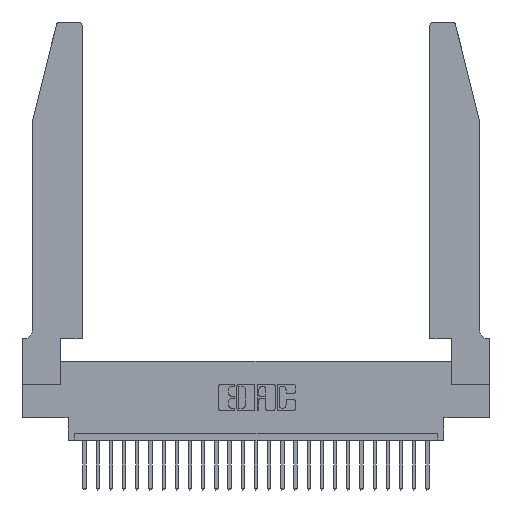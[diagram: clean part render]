
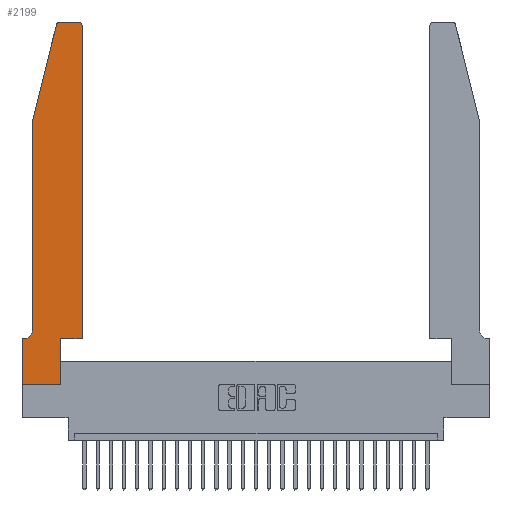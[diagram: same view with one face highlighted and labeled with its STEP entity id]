
A CAD part, top view. The second image highlights one B-rep face of the part: STEP entity #2199.
In plain terms, the highlighted planar face has unit normal (0, 0, 1).
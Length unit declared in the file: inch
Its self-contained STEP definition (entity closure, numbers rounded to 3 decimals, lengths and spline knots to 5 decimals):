
#155 = DIRECTION ( 'NONE',  ( 0., -1., 0. ) ) ;
#509 = VERTEX_POINT ( 'NONE', #19501 ) ;
#554 = CARTESIAN_POINT ( 'NONE',  ( 0., 0., 0.37 ) ) ;
#680 = DIRECTION ( 'NONE',  ( 1., 0., 0. ) ) ;
#775 = CARTESIAN_POINT ( 'NONE',  ( 0.4205, 2.72, 0.37 ) ) ;
#972 = VERTEX_POINT ( 'NONE', #25046 ) ;
#995 = ORIENTED_EDGE ( 'NONE', *, *, #1489, .T. ) ;
#1018 = LINE ( 'NONE', #25897, #25701 ) ;
#1271 = EDGE_CURVE ( 'NONE', #7114, #4585, #18498, .T. ) ;
#1489 = EDGE_CURVE ( 'NONE', #16377, #7114, #5650, .T. ) ;
#1569 = DIRECTION ( 'NONE',  ( -1., 0., 0. ) ) ;
#2199 = ADVANCED_FACE ( 'NONE', ( #20434 ), #17067, .T. ) ;
#2354 = CARTESIAN_POINT ( 'NONE',  ( 0.284, 2.75, 0.37 ) ) ;
#2361 = EDGE_CURVE ( 'NONE', #26980, #21348, #1018, .T. ) ;
#2566 = VECTOR ( 'NONE', #2654, 39.37008 ) ;
#2654 = DIRECTION ( 'NONE',  ( 1., 0., 0. ) ) ;
#2806 = DIRECTION ( 'NONE',  ( -0.239, -0.971, 0. ) ) ;
#2862 = EDGE_LOOP ( 'NONE', ( #25732, #5754, #26918, #20653, #3659, #995, #18751, #20708, #6925, #7870, #15923, #7170 ) ) ;
#2905 = CARTESIAN_POINT ( 'NONE',  ( 0.2865, 0.35, 0.37 ) ) ;
#2944 = DIRECTION ( 'NONE',  ( -1., 0., 0. ) ) ;
#3008 = VECTOR ( 'NONE', #6238, 39.37008 ) ;
#3348 = DIRECTION ( 'NONE',  ( 1., 0., 0. ) ) ;
#3659 = ORIENTED_EDGE ( 'NONE', *, *, #20299, .T. ) ;
#3690 = VECTOR ( 'NONE', #21560, 39.37008 ) ;
#4336 = CIRCLE ( 'NONE', #18900, 0.07 ) ;
#4585 = VERTEX_POINT ( 'NONE', #6536 ) ;
#4648 = VERTEX_POINT ( 'NONE', #2354 ) ;
#5087 = CARTESIAN_POINT ( 'NONE',  ( 0.0755, 0.42, 0.37 ) ) ;
#5310 = LINE ( 'NONE', #16421, #14200 ) ;
#5650 = LINE ( 'NONE', #9894, #16191 ) ;
#5754 = ORIENTED_EDGE ( 'NONE', *, *, #26614, .T. ) ;
#5980 = LINE ( 'NONE', #7974, #21845 ) ;
#6238 = DIRECTION ( 'NONE',  ( 0., 1., 0. ) ) ;
#6536 = CARTESIAN_POINT ( 'NONE',  ( 0., 0., 0.37 ) ) ;
#6803 = CARTESIAN_POINT ( 'NONE',  ( 0., 0., 0.37 ) ) ;
#6925 = ORIENTED_EDGE ( 'NONE', *, *, #19256, .T. ) ;
#7114 = VERTEX_POINT ( 'NONE', #18853 ) ;
#7170 = ORIENTED_EDGE ( 'NONE', *, *, #22832, .T. ) ;
#7190 = CARTESIAN_POINT ( 'NONE',  ( 0.4205, 2.75, 0.37 ) ) ;
#7447 = DIRECTION ( 'NONE',  ( 0., 0., 1. ) ) ;
#7870 = ORIENTED_EDGE ( 'NONE', *, *, #17607, .T. ) ;
#7974 = CARTESIAN_POINT ( 'NONE',  ( 0.2605, 2.75, 0.37 ) ) ;
#8051 = VERTEX_POINT ( 'NONE', #24405 ) ;
#9242 = DIRECTION ( 'NONE',  ( 0., 1., 0. ) ) ;
#9410 = EDGE_CURVE ( 'NONE', #21348, #13833, #5310, .T. ) ;
#9644 = VERTEX_POINT ( 'NONE', #16346 ) ;
#9894 = CARTESIAN_POINT ( 'NONE',  ( 0.0755, 0.35, 0.37 ) ) ;
#10034 = AXIS2_PLACEMENT_3D ( 'NONE', #14746, #19179, #21119 ) ;
#10352 = CARTESIAN_POINT ( 'NONE',  ( 0.25487, 2.72718, 0.37 ) ) ;
#10567 = CARTESIAN_POINT ( 'NONE',  ( 0.4505, 0.35, 0.37 ) ) ;
#10781 = CIRCLE ( 'NONE', #16338, 0.03 ) ;
#12180 = DIRECTION ( 'NONE',  ( -1., 0., 0. ) ) ;
#13404 = CARTESIAN_POINT ( 'NONE',  ( 0.0055, 0.42, 0.37 ) ) ;
#13833 = VERTEX_POINT ( 'NONE', #5087 ) ;
#13923 = EDGE_CURVE ( 'NONE', #509, #9644, #17154, .T. ) ;
#14200 = VECTOR ( 'NONE', #155, 39.37008 ) ;
#14704 = CARTESIAN_POINT ( 'NONE',  ( 0.0755, 2., 0.37 ) ) ;
#14746 = CARTESIAN_POINT ( 'NONE',  ( 0., 0.35, 0.37 ) ) ;
#15484 = DIRECTION ( 'NONE',  ( 0., 0., 1. ) ) ;
#15545 = DIRECTION ( 'NONE',  ( 0., 0., -1. ) ) ;
#15678 = VECTOR ( 'NONE', #26345, 39.37008 ) ;
#15923 = ORIENTED_EDGE ( 'NONE', *, *, #13923, .T. ) ;
#16191 = VECTOR ( 'NONE', #12180, 39.37008 ) ;
#16338 = AXIS2_PLACEMENT_3D ( 'NONE', #24414, #7447, #3348 ) ;
#16346 = CARTESIAN_POINT ( 'NONE',  ( 0.4505, 2.72, 0.37 ) ) ;
#16377 = VERTEX_POINT ( 'NONE', #25798 ) ;
#16421 = CARTESIAN_POINT ( 'NONE',  ( 0.0755, 2., 0.37 ) ) ;
#17067 = PLANE ( 'NONE',  #10034 ) ;
#17154 = LINE ( 'NONE', #10567, #3008 ) ;
#17607 = EDGE_CURVE ( 'NONE', #8051, #509, #24248, .T. ) ;
#18498 = LINE ( 'NONE', #6803, #3690 ) ;
#18751 = ORIENTED_EDGE ( 'NONE', *, *, #1271, .T. ) ;
#18853 = CARTESIAN_POINT ( 'NONE',  ( 0., 0.35, 0.37 ) ) ;
#18900 = AXIS2_PLACEMENT_3D ( 'NONE', #13404, #15545, #2944 ) ;
#19179 = DIRECTION ( 'NONE',  ( 0., 0., 1. ) ) ;
#19256 = EDGE_CURVE ( 'NONE', #972, #8051, #25141, .T. ) ;
#19501 = CARTESIAN_POINT ( 'NONE',  ( 0.4505, 0.35, 0.37 ) ) ;
#19563 = CARTESIAN_POINT ( 'NONE',  ( 0.4505, 0.35, 0.37 ) ) ;
#20194 = CIRCLE ( 'NONE', #26493, 0.03 ) ;
#20299 = EDGE_CURVE ( 'NONE', #13833, #16377, #4336, .T. ) ;
#20434 = FACE_OUTER_BOUND ( 'NONE', #2862, .T. ) ;
#20653 = ORIENTED_EDGE ( 'NONE', *, *, #9410, .T. ) ;
#20708 = ORIENTED_EDGE ( 'NONE', *, *, #25956, .T. ) ;
#21119 = DIRECTION ( 'NONE',  ( 1., 0., 0. ) ) ;
#21348 = VERTEX_POINT ( 'NONE', #14704 ) ;
#21560 = DIRECTION ( 'NONE',  ( 0., -1., 0. ) ) ;
#21845 = VECTOR ( 'NONE', #1569, 39.37008 ) ;
#22832 = EDGE_CURVE ( 'NONE', #9644, #26547, #20194, .T. ) ;
#23176 = EDGE_CURVE ( 'NONE', #26547, #4648, #5980, .T. ) ;
#24248 = LINE ( 'NONE', #19563, #15678 ) ;
#24405 = CARTESIAN_POINT ( 'NONE',  ( 0.2865, 0.35, 0.37 ) ) ;
#24414 = CARTESIAN_POINT ( 'NONE',  ( 0.284, 2.72, 0.37 ) ) ;
#25046 = CARTESIAN_POINT ( 'NONE',  ( 0.2865, 0., 0.37 ) ) ;
#25141 = LINE ( 'NONE', #2905, #25463 ) ;
#25297 = LINE ( 'NONE', #554, #2566 ) ;
#25463 = VECTOR ( 'NONE', #9242, 39.37008 ) ;
#25701 = VECTOR ( 'NONE', #2806, 39.37008 ) ;
#25732 = ORIENTED_EDGE ( 'NONE', *, *, #23176, .T. ) ;
#25798 = CARTESIAN_POINT ( 'NONE',  ( 0.0055, 0.35, 0.37 ) ) ;
#25897 = CARTESIAN_POINT ( 'NONE',  ( 0.0755, 2., 0.37 ) ) ;
#25956 = EDGE_CURVE ( 'NONE', #4585, #972, #25297, .T. ) ;
#26345 = DIRECTION ( 'NONE',  ( 1., 0., 0. ) ) ;
#26493 = AXIS2_PLACEMENT_3D ( 'NONE', #775, #15484, #680 ) ;
#26547 = VERTEX_POINT ( 'NONE', #7190 ) ;
#26614 = EDGE_CURVE ( 'NONE', #4648, #26980, #10781, .T. ) ;
#26918 = ORIENTED_EDGE ( 'NONE', *, *, #2361, .T. ) ;
#26980 = VERTEX_POINT ( 'NONE', #10352 ) ;
